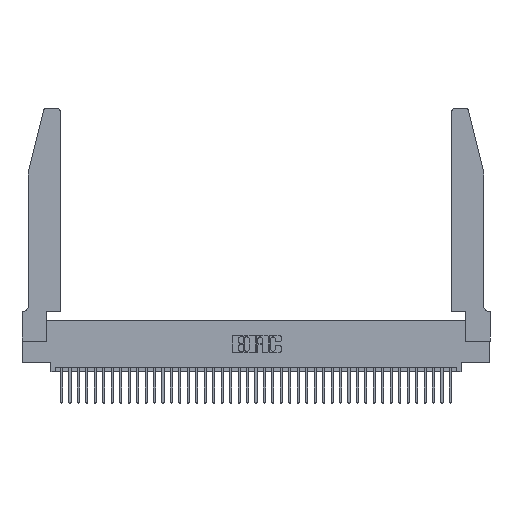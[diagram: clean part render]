
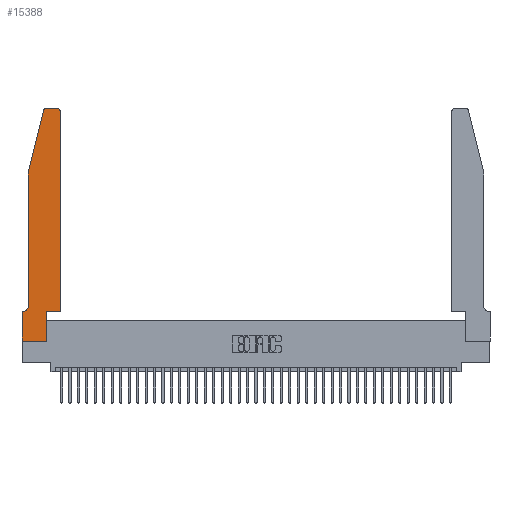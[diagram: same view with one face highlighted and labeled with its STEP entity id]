
A CAD part, top view. The second image highlights one B-rep face of the part: STEP entity #15388.
In plain terms, the highlighted planar face has unit normal (0, 0, 1).
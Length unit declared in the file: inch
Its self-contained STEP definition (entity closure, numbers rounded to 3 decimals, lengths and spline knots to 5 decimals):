
#1062 = VERTEX_POINT ( 'NONE', #23332 ) ;
#1993 = ORIENTED_EDGE ( 'NONE', *, *, #20082, .T. ) ;
#4566 = CARTESIAN_POINT ( 'NONE',  ( 0., 0., 0.37 ) ) ;
#4614 = CARTESIAN_POINT ( 'NONE',  ( 0.2865, 0.35, 0.37 ) ) ;
#5625 = CARTESIAN_POINT ( 'NONE',  ( 0.0055, 0.42, 0.37 ) ) ;
#6043 = ORIENTED_EDGE ( 'NONE', *, *, #38586, .T. ) ;
#6107 = VECTOR ( 'NONE', #28477, 39.37008 ) ;
#6560 = ORIENTED_EDGE ( 'NONE', *, *, #28028, .T. ) ;
#7368 = EDGE_CURVE ( 'NONE', #9247, #28498, #37496, .T. ) ;
#7595 = CARTESIAN_POINT ( 'NONE',  ( 0.0755, 0.35, 0.37 ) ) ;
#8841 = DIRECTION ( 'NONE',  ( -1., 0., 0. ) ) ;
#8941 = EDGE_CURVE ( 'NONE', #19378, #28884, #39839, .T. ) ;
#9031 = ORIENTED_EDGE ( 'NONE', *, *, #10534, .T. ) ;
#9153 = LINE ( 'NONE', #23588, #25067 ) ;
#9247 = VERTEX_POINT ( 'NONE', #4614 ) ;
#9363 = CARTESIAN_POINT ( 'NONE',  ( 0.284, 2.75, 0.37 ) ) ;
#9461 = EDGE_CURVE ( 'NONE', #1062, #11162, #21966, .T. ) ;
#9825 = LINE ( 'NONE', #18008, #34165 ) ;
#10147 = VECTOR ( 'NONE', #10796, 39.37008 ) ;
#10165 = VERTEX_POINT ( 'NONE', #21839 ) ;
#10534 = EDGE_CURVE ( 'NONE', #26129, #19378, #34789, .T. ) ;
#10643 = AXIS2_PLACEMENT_3D ( 'NONE', #5625, #27900, #8841 ) ;
#10680 = PLANE ( 'NONE',  #39810 ) ;
#10796 = DIRECTION ( 'NONE',  ( -1., 0., 0. ) ) ;
#11162 = VERTEX_POINT ( 'NONE', #29909 ) ;
#12826 = CARTESIAN_POINT ( 'NONE',  ( 0.25487, 2.72718, 0.37 ) ) ;
#13180 = CARTESIAN_POINT ( 'NONE',  ( 0.0755, 2., 0.37 ) ) ;
#13245 = EDGE_CURVE ( 'NONE', #10165, #23221, #38507, .T. ) ;
#13918 = DIRECTION ( 'NONE',  ( 0., 0., 1. ) ) ;
#13950 = CARTESIAN_POINT ( 'NONE',  ( 0., 0., 0.37 ) ) ;
#14504 = CARTESIAN_POINT ( 'NONE',  ( 0.2605, 2.75, 0.37 ) ) ;
#14716 = DIRECTION ( 'NONE',  ( 0., -1., 0. ) ) ;
#15064 = CARTESIAN_POINT ( 'NONE',  ( 0.2865, 0., 0.37 ) ) ;
#15388 = ADVANCED_FACE ( 'NONE', ( #30478 ), #10680, .T. ) ;
#16044 = CARTESIAN_POINT ( 'NONE',  ( 0.0755, 2., 0.37 ) ) ;
#16052 = VECTOR ( 'NONE', #16246, 39.37008 ) ;
#16246 = DIRECTION ( 'NONE',  ( -0.239, -0.971, 0. ) ) ;
#16923 = VECTOR ( 'NONE', #32957, 39.37008 ) ;
#17420 = VECTOR ( 'NONE', #14716, 39.37008 ) ;
#17647 = CIRCLE ( 'NONE', #39132, 0.03 ) ;
#18006 = ORIENTED_EDGE ( 'NONE', *, *, #13245, .T. ) ;
#18008 = CARTESIAN_POINT ( 'NONE',  ( 0.2865, 0.35, 0.37 ) ) ;
#18096 = CARTESIAN_POINT ( 'NONE',  ( 0.284, 2.72, 0.37 ) ) ;
#18217 = DIRECTION ( 'NONE',  ( 0., 0., 1. ) ) ;
#18405 = LINE ( 'NONE', #24159, #17420 ) ;
#18962 = ORIENTED_EDGE ( 'NONE', *, *, #7368, .T. ) ;
#19378 = VERTEX_POINT ( 'NONE', #4566 ) ;
#19678 = CARTESIAN_POINT ( 'NONE',  ( 0.4505, 2.72, 0.37 ) ) ;
#20033 = EDGE_CURVE ( 'NONE', #11162, #26129, #27077, .T. ) ;
#20082 = EDGE_CURVE ( 'NONE', #28498, #38276, #9153, .T. ) ;
#20498 = CARTESIAN_POINT ( 'NONE',  ( 0.4505, 0.35, 0.37 ) ) ;
#21273 = DIRECTION ( 'NONE',  ( 1., 0., 0. ) ) ;
#21839 = CARTESIAN_POINT ( 'NONE',  ( 0.4205, 2.75, 0.37 ) ) ;
#21966 = CIRCLE ( 'NONE', #10643, 0.07 ) ;
#22346 = EDGE_CURVE ( 'NONE', #33161, #1062, #18405, .T. ) ;
#23221 = VERTEX_POINT ( 'NONE', #9363 ) ;
#23332 = CARTESIAN_POINT ( 'NONE',  ( 0.0755, 0.42, 0.37 ) ) ;
#23588 = CARTESIAN_POINT ( 'NONE',  ( 0.4505, 0.35, 0.37 ) ) ;
#24159 = CARTESIAN_POINT ( 'NONE',  ( 0.0755, 2., 0.37 ) ) ;
#24169 = VERTEX_POINT ( 'NONE', #12826 ) ;
#24261 = AXIS2_PLACEMENT_3D ( 'NONE', #18096, #40241, #21273 ) ;
#25067 = VECTOR ( 'NONE', #26799, 39.37008 ) ;
#25243 = CARTESIAN_POINT ( 'NONE',  ( 0., 0., 0.37 ) ) ;
#26129 = VERTEX_POINT ( 'NONE', #38026 ) ;
#26799 = DIRECTION ( 'NONE',  ( 0., 1., 0. ) ) ;
#27077 = LINE ( 'NONE', #7595, #10147 ) ;
#27900 = DIRECTION ( 'NONE',  ( 0., 0., -1. ) ) ;
#28028 = EDGE_CURVE ( 'NONE', #24169, #33161, #32946, .T. ) ;
#28144 = VECTOR ( 'NONE', #30128, 39.37008 ) ;
#28477 = DIRECTION ( 'NONE',  ( 1., 0., 0. ) ) ;
#28498 = VERTEX_POINT ( 'NONE', #35329 ) ;
#28884 = VERTEX_POINT ( 'NONE', #15064 ) ;
#29909 = CARTESIAN_POINT ( 'NONE',  ( 0.0055, 0.35, 0.37 ) ) ;
#30128 = DIRECTION ( 'NONE',  ( 1., 0., 0. ) ) ;
#30302 = EDGE_CURVE ( 'NONE', #23221, #24169, #33719, .T. ) ;
#30478 = FACE_OUTER_BOUND ( 'NONE', #37189, .T. ) ;
#31417 = ORIENTED_EDGE ( 'NONE', *, *, #8941, .T. ) ;
#32132 = VECTOR ( 'NONE', #36644, 39.37008 ) ;
#32895 = ORIENTED_EDGE ( 'NONE', *, *, #40237, .T. ) ;
#32935 = CARTESIAN_POINT ( 'NONE',  ( 0., 0.35, 0.37 ) ) ;
#32946 = LINE ( 'NONE', #13180, #16052 ) ;
#32957 = DIRECTION ( 'NONE',  ( 0., -1., 0. ) ) ;
#33161 = VERTEX_POINT ( 'NONE', #16044 ) ;
#33719 = CIRCLE ( 'NONE', #24261, 0.03 ) ;
#33903 = ORIENTED_EDGE ( 'NONE', *, *, #30302, .T. ) ;
#34165 = VECTOR ( 'NONE', #40152, 39.37008 ) ;
#34369 = ORIENTED_EDGE ( 'NONE', *, *, #20033, .T. ) ;
#34789 = LINE ( 'NONE', #13950, #16923 ) ;
#35329 = CARTESIAN_POINT ( 'NONE',  ( 0.4505, 0.35, 0.37 ) ) ;
#36061 = DIRECTION ( 'NONE',  ( 1., 0., 0. ) ) ;
#36340 = ORIENTED_EDGE ( 'NONE', *, *, #9461, .T. ) ;
#36644 = DIRECTION ( 'NONE',  ( -1., 0., 0. ) ) ;
#37184 = CARTESIAN_POINT ( 'NONE',  ( 0.4205, 2.72, 0.37 ) ) ;
#37189 = EDGE_LOOP ( 'NONE', ( #18006, #33903, #6560, #37311, #36340, #34369, #9031, #31417, #6043, #18962, #1993, #32895 ) ) ;
#37311 = ORIENTED_EDGE ( 'NONE', *, *, #22346, .T. ) ;
#37496 = LINE ( 'NONE', #20498, #28144 ) ;
#38026 = CARTESIAN_POINT ( 'NONE',  ( 0., 0.35, 0.37 ) ) ;
#38276 = VERTEX_POINT ( 'NONE', #19678 ) ;
#38507 = LINE ( 'NONE', #14504, #32132 ) ;
#38586 = EDGE_CURVE ( 'NONE', #28884, #9247, #9825, .T. ) ;
#39132 = AXIS2_PLACEMENT_3D ( 'NONE', #37184, #18217, #40358 ) ;
#39810 = AXIS2_PLACEMENT_3D ( 'NONE', #32935, #13918, #36061 ) ;
#39839 = LINE ( 'NONE', #25243, #6107 ) ;
#40152 = DIRECTION ( 'NONE',  ( 0., 1., 0. ) ) ;
#40237 = EDGE_CURVE ( 'NONE', #38276, #10165, #17647, .T. ) ;
#40241 = DIRECTION ( 'NONE',  ( 0., 0., 1. ) ) ;
#40358 = DIRECTION ( 'NONE',  ( 1., 0., 0. ) ) ;
